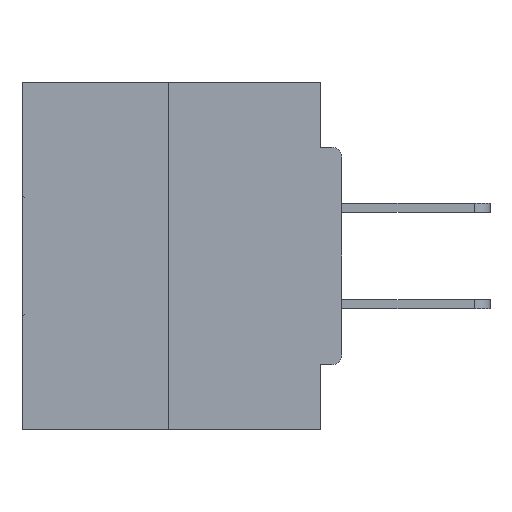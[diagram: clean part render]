
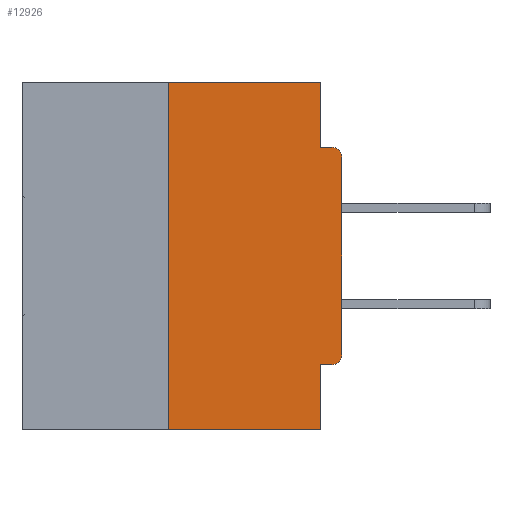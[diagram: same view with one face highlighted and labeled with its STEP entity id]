
A CAD part, left-side view. The second image highlights one B-rep face of the part: STEP entity #12926.
In plain terms, the highlighted planar face has unit normal (-1, 0, 0).
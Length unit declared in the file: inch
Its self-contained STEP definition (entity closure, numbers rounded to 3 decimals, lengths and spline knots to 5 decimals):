
#320 = DIRECTION ( 'NONE',  ( 0., 0., 1. ) ) ;
#701 = CARTESIAN_POINT ( 'NONE',  ( 0., 0.031, -0.5 ) ) ;
#963 = VECTOR ( 'NONE', #31348, 39.37008 ) ;
#1224 = CARTESIAN_POINT ( 'NONE',  ( 0., 0.46, 0. ) ) ;
#2206 = CARTESIAN_POINT ( 'NONE',  ( 0., 0.25, 0. ) ) ;
#2250 = ORIENTED_EDGE ( 'NONE', *, *, #26488, .T. ) ;
#3042 = EDGE_CURVE ( 'NONE', #7121, #5691, #21377, .T. ) ;
#3677 = ORIENTED_EDGE ( 'NONE', *, *, #34269, .T. ) ;
#3898 = VERTEX_POINT ( 'NONE', #35538 ) ;
#4026 = CARTESIAN_POINT ( 'NONE',  ( 0., 0., -0.0935 ) ) ;
#4526 = CARTESIAN_POINT ( 'NONE',  ( 0., 0.46, -0.5 ) ) ;
#5161 = LINE ( 'NONE', #4526, #38114 ) ;
#5691 = VERTEX_POINT ( 'NONE', #36194 ) ;
#6199 = LINE ( 'NONE', #701, #23456 ) ;
#6574 = FACE_OUTER_BOUND ( 'NONE', #11012, .T. ) ;
#7078 = DIRECTION ( 'NONE',  ( 0., 0., -1. ) ) ;
#7121 = VERTEX_POINT ( 'NONE', #40961 ) ;
#7728 = VERTEX_POINT ( 'NONE', #22481 ) ;
#8484 = PLANE ( 'NONE',  #39645 ) ;
#8624 = DIRECTION ( 'NONE',  ( 1., 0., 0. ) ) ;
#8869 = LINE ( 'NONE', #4026, #26133 ) ;
#9179 = DIRECTION ( 'NONE',  ( 0., 0., -1. ) ) ;
#9234 = EDGE_CURVE ( 'NONE', #26635, #33491, #6199, .T. ) ;
#9278 = VERTEX_POINT ( 'NONE', #16545 ) ;
#10964 = DIRECTION ( 'NONE',  ( 0., -1., 0. ) ) ;
#11012 = EDGE_LOOP ( 'NONE', ( #33001, #16304, #3677, #30508, #23059, #27451, #2250, #20730, #18867, #25341 ) ) ;
#12166 = AXIS2_PLACEMENT_3D ( 'NONE', #14151, #14006, #7078 ) ;
#12926 = ADVANCED_FACE ( 'NONE', ( #6574 ), #8484, .F. ) ;
#13947 = CIRCLE ( 'NONE', #12166, 0.015 ) ;
#14006 = DIRECTION ( 'NONE',  ( -1., 0., 0. ) ) ;
#14151 = CARTESIAN_POINT ( 'NONE',  ( 0., 0.015, -0.3915 ) ) ;
#15364 = EDGE_CURVE ( 'NONE', #5691, #3898, #8869, .T. ) ;
#15578 = CARTESIAN_POINT ( 'NONE',  ( 0., 0.25, 0. ) ) ;
#16304 = ORIENTED_EDGE ( 'NONE', *, *, #36473, .F. ) ;
#16545 = CARTESIAN_POINT ( 'NONE',  ( 0., 0., -0.1085 ) ) ;
#16589 = CARTESIAN_POINT ( 'NONE',  ( 0., 0., 0. ) ) ;
#16635 = LINE ( 'NONE', #1224, #34967 ) ;
#18862 = DIRECTION ( 'NONE',  ( -1., 0., 0. ) ) ;
#18867 = ORIENTED_EDGE ( 'NONE', *, *, #15364, .F. ) ;
#18876 = DIRECTION ( 'NONE',  ( 0., 0., -1. ) ) ;
#19225 = CARTESIAN_POINT ( 'NONE',  ( 0., 0.031, -0.5 ) ) ;
#19949 = EDGE_CURVE ( 'NONE', #22205, #27276, #13947, .T. ) ;
#20730 = ORIENTED_EDGE ( 'NONE', *, *, #22603, .T. ) ;
#21186 = CARTESIAN_POINT ( 'NONE',  ( 0., 0., -0.4065 ) ) ;
#21296 = LINE ( 'NONE', #21186, #963 ) ;
#21377 = LINE ( 'NONE', #38528, #30980 ) ;
#22205 = VERTEX_POINT ( 'NONE', #27365 ) ;
#22411 = VECTOR ( 'NONE', #320, 39.37008 ) ;
#22481 = CARTESIAN_POINT ( 'NONE',  ( 0., 0.25, -0.5 ) ) ;
#22603 = EDGE_CURVE ( 'NONE', #9278, #3898, #29483, .T. ) ;
#23059 = ORIENTED_EDGE ( 'NONE', *, *, #23394, .F. ) ;
#23257 = VECTOR ( 'NONE', #41888, 39.37008 ) ;
#23394 = EDGE_CURVE ( 'NONE', #22205, #26635, #21296, .T. ) ;
#23456 = VECTOR ( 'NONE', #36091, 39.37008 ) ;
#25341 = ORIENTED_EDGE ( 'NONE', *, *, #3042, .F. ) ;
#25822 = CARTESIAN_POINT ( 'NONE',  ( 0., 0.015, -0.1085 ) ) ;
#26133 = VECTOR ( 'NONE', #36446, 39.37008 ) ;
#26488 = EDGE_CURVE ( 'NONE', #27276, #9278, #31056, .T. ) ;
#26635 = VERTEX_POINT ( 'NONE', #36839 ) ;
#27276 = VERTEX_POINT ( 'NONE', #28064 ) ;
#27365 = CARTESIAN_POINT ( 'NONE',  ( 0., 0.015, -0.4065 ) ) ;
#27451 = ORIENTED_EDGE ( 'NONE', *, *, #19949, .T. ) ;
#28064 = CARTESIAN_POINT ( 'NONE',  ( 0., 0., -0.3915 ) ) ;
#28207 = VERTEX_POINT ( 'NONE', #2206 ) ;
#29483 = CIRCLE ( 'NONE', #41505, 0.015 ) ;
#30378 = LINE ( 'NONE', #15578, #23257 ) ;
#30437 = DIRECTION ( 'NONE',  ( 0., -1., 0. ) ) ;
#30508 = ORIENTED_EDGE ( 'NONE', *, *, #9234, .F. ) ;
#30980 = VECTOR ( 'NONE', #18876, 39.37008 ) ;
#31056 = LINE ( 'NONE', #16589, #22411 ) ;
#31348 = DIRECTION ( 'NONE',  ( 0., 1., 0. ) ) ;
#33001 = ORIENTED_EDGE ( 'NONE', *, *, #35963, .F. ) ;
#33491 = VERTEX_POINT ( 'NONE', #19225 ) ;
#34017 = DIRECTION ( 'NONE',  ( 0., 0., -1. ) ) ;
#34269 = EDGE_CURVE ( 'NONE', #7728, #33491, #5161, .T. ) ;
#34967 = VECTOR ( 'NONE', #10964, 39.37008 ) ;
#35538 = CARTESIAN_POINT ( 'NONE',  ( 0., 0.015, -0.0935 ) ) ;
#35963 = EDGE_CURVE ( 'NONE', #28207, #7121, #16635, .T. ) ;
#36091 = DIRECTION ( 'NONE',  ( 0., 0., -1. ) ) ;
#36194 = CARTESIAN_POINT ( 'NONE',  ( 0., 0.031, -0.0935 ) ) ;
#36446 = DIRECTION ( 'NONE',  ( 0., -1., 0. ) ) ;
#36473 = EDGE_CURVE ( 'NONE', #7728, #28207, #30378, .T. ) ;
#36839 = CARTESIAN_POINT ( 'NONE',  ( 0., 0.031, -0.4065 ) ) ;
#37698 = CARTESIAN_POINT ( 'NONE',  ( 0., 0.46, 0. ) ) ;
#38114 = VECTOR ( 'NONE', #30437, 39.37008 ) ;
#38528 = CARTESIAN_POINT ( 'NONE',  ( 0., 0.031, 0. ) ) ;
#39645 = AXIS2_PLACEMENT_3D ( 'NONE', #37698, #8624, #34017 ) ;
#40961 = CARTESIAN_POINT ( 'NONE',  ( 0., 0.031, 0. ) ) ;
#41505 = AXIS2_PLACEMENT_3D ( 'NONE', #25822, #18862, #9179 ) ;
#41888 = DIRECTION ( 'NONE',  ( 0., 0., 1. ) ) ;
